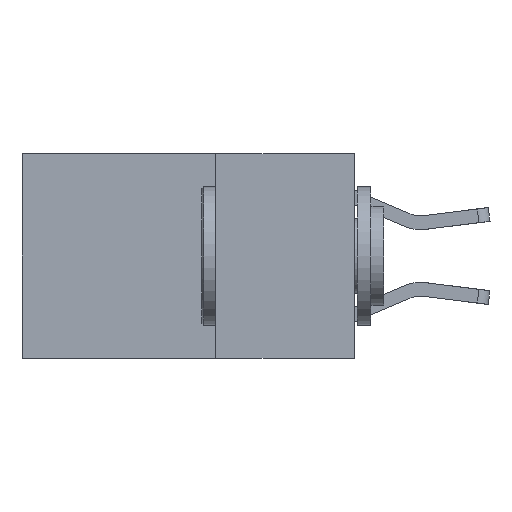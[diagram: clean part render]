
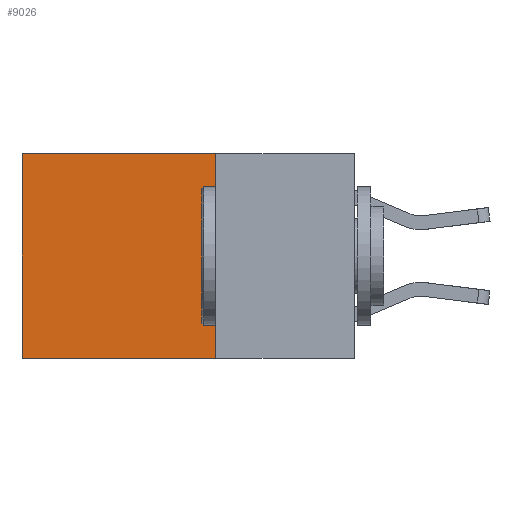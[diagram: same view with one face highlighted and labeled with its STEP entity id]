
A CAD part, left-side view. The second image highlights one B-rep face of the part: STEP entity #9026.
In plain terms, the highlighted planar face has unit normal (-1, 0, 0).
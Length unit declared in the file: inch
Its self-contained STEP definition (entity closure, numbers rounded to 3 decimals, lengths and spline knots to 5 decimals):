
#21 = LINE ( 'NONE', #1322, #9703 ) ;
#267 = AXIS2_PLACEMENT_3D ( 'NONE', #6225, #8907, #3305 ) ;
#327 = CARTESIAN_POINT ( 'NONE',  ( 0.2625, 0.6, 0. ) ) ;
#983 = VERTEX_POINT ( 'NONE', #6319 ) ;
#1213 = ORIENTED_EDGE ( 'NONE', *, *, #2888, .T. ) ;
#1322 = CARTESIAN_POINT ( 'NONE',  ( 0.2625, 0.6, 0. ) ) ;
#1766 = EDGE_CURVE ( 'NONE', #9527, #6630, #3936, .T. ) ;
#2293 = PLANE ( 'NONE',  #267 ) ;
#2365 = DIRECTION ( 'NONE',  ( 0., 0., -1. ) ) ;
#2714 = DIRECTION ( 'NONE',  ( 0., 0., -1. ) ) ;
#2888 = EDGE_CURVE ( 'NONE', #6630, #983, #21, .T. ) ;
#2910 = LINE ( 'NONE', #10155, #7712 ) ;
#3104 = EDGE_CURVE ( 'NONE', #10189, #983, #5757, .T. ) ;
#3136 = VECTOR ( 'NONE', #4812, 39.37008 ) ;
#3305 = DIRECTION ( 'NONE',  ( 0., 0., -1. ) ) ;
#3891 = ORIENTED_EDGE ( 'NONE', *, *, #1766, .T. ) ;
#3936 = LINE ( 'NONE', #5056, #11133 ) ;
#4812 = DIRECTION ( 'NONE',  ( 0., 1., 0. ) ) ;
#5056 = CARTESIAN_POINT ( 'NONE',  ( 0.2625, 0.25, 0. ) ) ;
#5757 = LINE ( 'NONE', #9397, #3136 ) ;
#6225 = CARTESIAN_POINT ( 'NONE',  ( 0.2625, 0.25, 0. ) ) ;
#6319 = CARTESIAN_POINT ( 'NONE',  ( 0.2625, 0.6, -0.37 ) ) ;
#6375 = EDGE_CURVE ( 'NONE', #9527, #10189, #2910, .T. ) ;
#6630 = VERTEX_POINT ( 'NONE', #327 ) ;
#7233 = ORIENTED_EDGE ( 'NONE', *, *, #3104, .F. ) ;
#7483 = EDGE_LOOP ( 'NONE', ( #1213, #7233, #11474, #3891 ) ) ;
#7526 = CARTESIAN_POINT ( 'NONE',  ( 0.2625, 0.25, -0.37 ) ) ;
#7712 = VECTOR ( 'NONE', #2714, 39.37008 ) ;
#8746 = CARTESIAN_POINT ( 'NONE',  ( 0.2625, 0.25, 0. ) ) ;
#8907 = DIRECTION ( 'NONE',  ( 1., 0., 0. ) ) ;
#9026 = ADVANCED_FACE ( 'NONE', ( #10624 ), #2293, .F. ) ;
#9397 = CARTESIAN_POINT ( 'NONE',  ( 0.2625, 0.25, -0.37 ) ) ;
#9527 = VERTEX_POINT ( 'NONE', #8746 ) ;
#9703 = VECTOR ( 'NONE', #2365, 39.37008 ) ;
#10155 = CARTESIAN_POINT ( 'NONE',  ( 0.2625, 0.25, 0. ) ) ;
#10189 = VERTEX_POINT ( 'NONE', #7526 ) ;
#10466 = DIRECTION ( 'NONE',  ( 0., 1., 0. ) ) ;
#10624 = FACE_OUTER_BOUND ( 'NONE', #7483, .T. ) ;
#11133 = VECTOR ( 'NONE', #10466, 39.37008 ) ;
#11474 = ORIENTED_EDGE ( 'NONE', *, *, #6375, .F. ) ;
